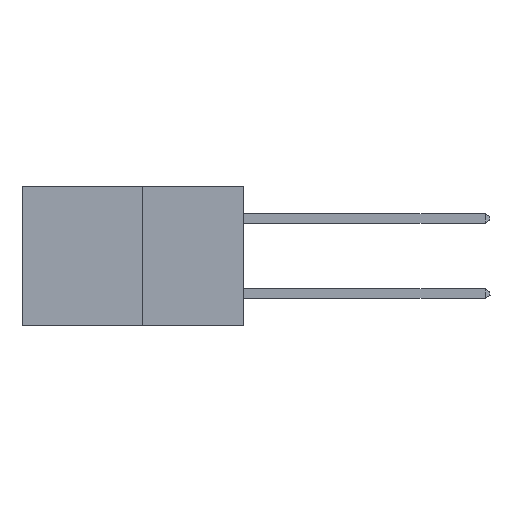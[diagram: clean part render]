
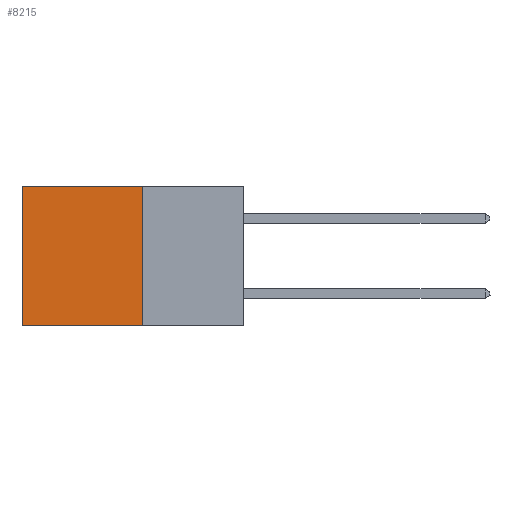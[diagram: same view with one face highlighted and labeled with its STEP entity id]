
A CAD part, left-side view. The second image highlights one B-rep face of the part: STEP entity #8215.
In plain terms, the highlighted planar face has unit normal (-1, 0, 0).
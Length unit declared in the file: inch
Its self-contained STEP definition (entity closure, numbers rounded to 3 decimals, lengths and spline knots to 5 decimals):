
#213 = AXIS2_PLACEMENT_3D ( 'NONE', #6930, #6911, #6892 ) ;
#218 = VERTEX_POINT ( 'NONE', #473 ) ;
#247 = CARTESIAN_POINT ( 'NONE',  ( 0.277, 0.59, 0. ) ) ;
#473 = CARTESIAN_POINT ( 'NONE',  ( 0.277, 0.59, -0.37 ) ) ;
#547 = VECTOR ( 'NONE', #2492, 39.37008 ) ;
#1205 = VERTEX_POINT ( 'NONE', #8788 ) ;
#2248 = VERTEX_POINT ( 'NONE', #247 ) ;
#2404 = VECTOR ( 'NONE', #6025, 39.37008 ) ;
#2492 = DIRECTION ( 'NONE',  ( 0., 0., -1. ) ) ;
#2669 = DIRECTION ( 'NONE',  ( 0., 1., 0. ) ) ;
#2700 = CARTESIAN_POINT ( 'NONE',  ( 0.277, 0.27, 0. ) ) ;
#4492 = LINE ( 'NONE', #6181, #2404 ) ;
#4734 = ORIENTED_EDGE ( 'NONE', *, *, #5615, .T. ) ;
#5210 = LINE ( 'NONE', #6220, #8700 ) ;
#5615 = EDGE_CURVE ( 'NONE', #2248, #218, #8463, .T. ) ;
#6005 = EDGE_CURVE ( 'NONE', #8426, #1205, #5210, .T. ) ;
#6025 = DIRECTION ( 'NONE',  ( 0., 1., 0. ) ) ;
#6040 = CARTESIAN_POINT ( 'NONE',  ( 0.277, 0.27, 0. ) ) ;
#6181 = CARTESIAN_POINT ( 'NONE',  ( 0.277, 0.27, -0.37 ) ) ;
#6220 = CARTESIAN_POINT ( 'NONE',  ( 0.277, 0.27, -0.37 ) ) ;
#6327 = DIRECTION ( 'NONE',  ( 0., 0., -1. ) ) ;
#6683 = EDGE_CURVE ( 'NONE', #1205, #218, #4492, .T. ) ;
#6892 = DIRECTION ( 'NONE',  ( 0., 0., -1. ) ) ;
#6911 = DIRECTION ( 'NONE',  ( 1., 0., 0. ) ) ;
#6930 = CARTESIAN_POINT ( 'NONE',  ( 0.277, 0.27, -0.37 ) ) ;
#6950 = PLANE ( 'NONE',  #213 ) ;
#7334 = ORIENTED_EDGE ( 'NONE', *, *, #6005, .F. ) ;
#7531 = ORIENTED_EDGE ( 'NONE', *, *, #9169, .T. ) ;
#8215 = ADVANCED_FACE ( 'NONE', ( #9404 ), #6950, .F. ) ;
#8267 = EDGE_LOOP ( 'NONE', ( #4734, #8498, #7334, #7531 ) ) ;
#8417 = VECTOR ( 'NONE', #2669, 39.37008 ) ;
#8426 = VERTEX_POINT ( 'NONE', #6040 ) ;
#8463 = LINE ( 'NONE', #8800, #547 ) ;
#8498 = ORIENTED_EDGE ( 'NONE', *, *, #6683, .F. ) ;
#8661 = LINE ( 'NONE', #2700, #8417 ) ;
#8700 = VECTOR ( 'NONE', #6327, 39.37008 ) ;
#8788 = CARTESIAN_POINT ( 'NONE',  ( 0.277, 0.27, -0.37 ) ) ;
#8800 = CARTESIAN_POINT ( 'NONE',  ( 0.277, 0.59, -0.37 ) ) ;
#9169 = EDGE_CURVE ( 'NONE', #8426, #2248, #8661, .T. ) ;
#9404 = FACE_OUTER_BOUND ( 'NONE', #8267, .T. ) ;
